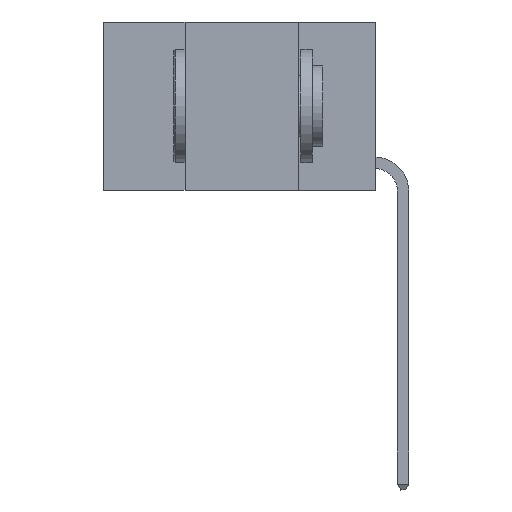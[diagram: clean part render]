
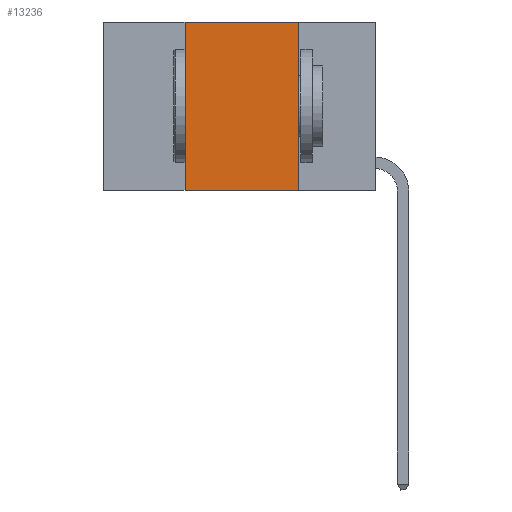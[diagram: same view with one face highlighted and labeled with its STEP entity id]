
A CAD part, left-side view. The second image highlights one B-rep face of the part: STEP entity #13236.
In plain terms, the highlighted planar face has unit normal (-1, 0, 0).
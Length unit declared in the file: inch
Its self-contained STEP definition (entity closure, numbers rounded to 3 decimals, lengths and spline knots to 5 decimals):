
#857 = VECTOR ( 'NONE', #12253, 39.37008 ) ;
#1188 = EDGE_CURVE ( 'NONE', #13322, #13267, #7635, .T. ) ;
#3774 = DIRECTION ( 'NONE',  ( 0., 0., 1. ) ) ;
#3989 = VECTOR ( 'NONE', #3774, 39.37008 ) ;
#4165 = DIRECTION ( 'NONE',  ( 0., -1., 0. ) ) ;
#4447 = FACE_OUTER_BOUND ( 'NONE', #8865, .T. ) ;
#4659 = CARTESIAN_POINT ( 'NONE',  ( 0., 0.6, 0. ) ) ;
#5805 = ORIENTED_EDGE ( 'NONE', *, *, #12087, .F. ) ;
#5891 = DIRECTION ( 'NONE',  ( 0., 0., -1. ) ) ;
#7511 = VECTOR ( 'NONE', #4165, 39.37008 ) ;
#7635 = LINE ( 'NONE', #12393, #857 ) ;
#8270 = VECTOR ( 'NONE', #9716, 39.37008 ) ;
#8535 = CARTESIAN_POINT ( 'NONE',  ( 0., 0.17, 0. ) ) ;
#8865 = EDGE_LOOP ( 'NONE', ( #5805, #8962, #12058, #9344 ) ) ;
#8921 = CARTESIAN_POINT ( 'NONE',  ( 0., 0.6, -0.37 ) ) ;
#8962 = ORIENTED_EDGE ( 'NONE', *, *, #1188, .F. ) ;
#9272 = VERTEX_POINT ( 'NONE', #14710 ) ;
#9344 = ORIENTED_EDGE ( 'NONE', *, *, #12302, .T. ) ;
#9470 = CARTESIAN_POINT ( 'NONE',  ( 0., 0.17, 0. ) ) ;
#9716 = DIRECTION ( 'NONE',  ( 0., 0., -1. ) ) ;
#9794 = CARTESIAN_POINT ( 'NONE',  ( 0., 0.42, 0. ) ) ;
#10370 = EDGE_CURVE ( 'NONE', #13713, #13322, #13384, .T. ) ;
#10645 = LINE ( 'NONE', #8921, #7511 ) ;
#10733 = CARTESIAN_POINT ( 'NONE',  ( 0., 0.42, 0. ) ) ;
#11433 = CARTESIAN_POINT ( 'NONE',  ( 0., 0.42, -0.37 ) ) ;
#12058 = ORIENTED_EDGE ( 'NONE', *, *, #10370, .F. ) ;
#12087 = EDGE_CURVE ( 'NONE', #13267, #9272, #14242, .T. ) ;
#12253 = DIRECTION ( 'NONE',  ( 0., -1., 0. ) ) ;
#12302 = EDGE_CURVE ( 'NONE', #13713, #9272, #10645, .T. ) ;
#12393 = CARTESIAN_POINT ( 'NONE',  ( 0., 0.6, 0. ) ) ;
#12411 = AXIS2_PLACEMENT_3D ( 'NONE', #4659, #12914, #5891 ) ;
#12864 = PLANE ( 'NONE',  #12411 ) ;
#12914 = DIRECTION ( 'NONE',  ( 1., 0., 0. ) ) ;
#13236 = ADVANCED_FACE ( 'NONE', ( #4447 ), #12864, .F. ) ;
#13267 = VERTEX_POINT ( 'NONE', #9470 ) ;
#13322 = VERTEX_POINT ( 'NONE', #10733 ) ;
#13384 = LINE ( 'NONE', #9794, #3989 ) ;
#13713 = VERTEX_POINT ( 'NONE', #11433 ) ;
#14242 = LINE ( 'NONE', #8535, #8270 ) ;
#14710 = CARTESIAN_POINT ( 'NONE',  ( 0., 0.17, -0.37 ) ) ;
